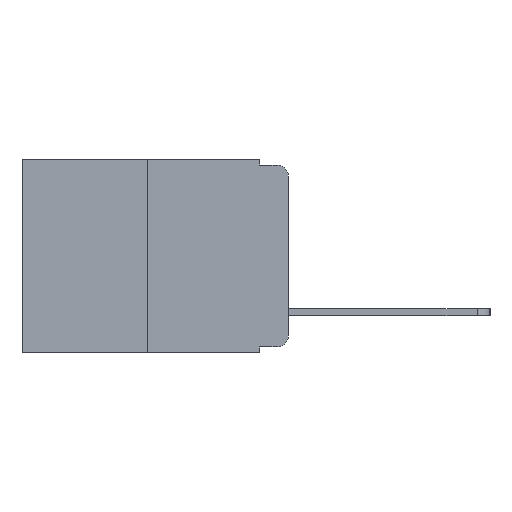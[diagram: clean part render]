
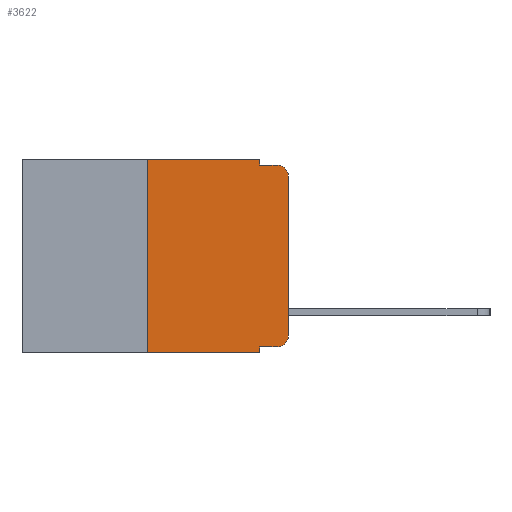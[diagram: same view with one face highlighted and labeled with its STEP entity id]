
A CAD part, left-side view. The second image highlights one B-rep face of the part: STEP entity #3622.
In plain terms, the highlighted planar face has unit normal (-1, 0, 0).
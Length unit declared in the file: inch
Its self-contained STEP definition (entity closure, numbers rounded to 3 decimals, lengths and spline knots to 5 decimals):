
#188 = LINE ( 'NONE', #12407, #15131 ) ;
#197 = CARTESIAN_POINT ( 'NONE',  ( 0., 0.02, -0.01 ) ) ;
#199 = ORIENTED_EDGE ( 'NONE', *, *, #7964, .T. ) ;
#202 = AXIS2_PLACEMENT_3D ( 'NONE', #255, #10537, #1770 ) ;
#255 = CARTESIAN_POINT ( 'NONE',  ( 0., 0.02, -0.03 ) ) ;
#1213 = EDGE_CURVE ( 'NONE', #17160, #12179, #15938, .T. ) ;
#1670 = DIRECTION ( 'NONE',  ( -1., 0., 0. ) ) ;
#1691 = EDGE_CURVE ( 'NONE', #12201, #5552, #12476, .T. ) ;
#1770 = DIRECTION ( 'NONE',  ( 0., 0., -1. ) ) ;
#1968 = ORIENTED_EDGE ( 'NONE', *, *, #8998, .F. ) ;
#2280 = ORIENTED_EDGE ( 'NONE', *, *, #17962, .T. ) ;
#2864 = EDGE_CURVE ( 'NONE', #15875, #12201, #16557, .T. ) ;
#3067 = DIRECTION ( 'NONE',  ( 0., -1., 0. ) ) ;
#3622 = ADVANCED_FACE ( 'NONE', ( #7149 ), #9745, .F. ) ;
#3859 = DIRECTION ( 'NONE',  ( 0., 0., -1. ) ) ;
#3867 = VERTEX_POINT ( 'NONE', #197 ) ;
#4126 = AXIS2_PLACEMENT_3D ( 'NONE', #13726, #9920, #9865 ) ;
#5187 = VECTOR ( 'NONE', #12238, 39.37008 ) ;
#5328 = VECTOR ( 'NONE', #7999, 39.37008 ) ;
#5380 = EDGE_CURVE ( 'NONE', #5552, #3867, #6384, .T. ) ;
#5424 = CARTESIAN_POINT ( 'NONE',  ( 0., 0.25, -0.343 ) ) ;
#5552 = VERTEX_POINT ( 'NONE', #9470 ) ;
#5699 = CARTESIAN_POINT ( 'NONE',  ( 0., 0.051, 0. ) ) ;
#5768 = ORIENTED_EDGE ( 'NONE', *, *, #1691, .F. ) ;
#5816 = CARTESIAN_POINT ( 'NONE',  ( 0., 0.02, -0.333 ) ) ;
#6181 = CARTESIAN_POINT ( 'NONE',  ( 0., 0.473, 0. ) ) ;
#6195 = ORIENTED_EDGE ( 'NONE', *, *, #9345, .T. ) ;
#6245 = ORIENTED_EDGE ( 'NONE', *, *, #5380, .F. ) ;
#6384 = LINE ( 'NONE', #17442, #13852 ) ;
#6517 = VERTEX_POINT ( 'NONE', #12123 ) ;
#6801 = CIRCLE ( 'NONE', #12951, 0.02 ) ;
#6941 = EDGE_LOOP ( 'NONE', ( #2280, #199, #6245, #5768, #10215, #1968, #10536, #10791, #6195, #10866 ) ) ;
#7149 = FACE_OUTER_BOUND ( 'NONE', #6941, .T. ) ;
#7195 = VERTEX_POINT ( 'NONE', #5816 ) ;
#7964 = EDGE_CURVE ( 'NONE', #17466, #3867, #17334, .T. ) ;
#7999 = DIRECTION ( 'NONE',  ( 0., -1., 0. ) ) ;
#8424 = LINE ( 'NONE', #9831, #15376 ) ;
#8998 = EDGE_CURVE ( 'NONE', #17160, #15875, #16871, .T. ) ;
#9116 = DIRECTION ( 'NONE',  ( 0., -1., 0. ) ) ;
#9194 = VERTEX_POINT ( 'NONE', #13927 ) ;
#9345 = EDGE_CURVE ( 'NONE', #9194, #7195, #14921, .T. ) ;
#9470 = CARTESIAN_POINT ( 'NONE',  ( 0., 0.051, -0.01 ) ) ;
#9745 = PLANE ( 'NONE',  #4126 ) ;
#9831 = CARTESIAN_POINT ( 'NONE',  ( 0., 0., 0. ) ) ;
#9865 = DIRECTION ( 'NONE',  ( 0., 0., -1. ) ) ;
#9920 = DIRECTION ( 'NONE',  ( 1., 0., 0. ) ) ;
#10076 = CARTESIAN_POINT ( 'NONE',  ( 0., 0.051, -0.333 ) ) ;
#10215 = ORIENTED_EDGE ( 'NONE', *, *, #2864, .F. ) ;
#10444 = CARTESIAN_POINT ( 'NONE',  ( 0., 0.02, -0.313 ) ) ;
#10536 = ORIENTED_EDGE ( 'NONE', *, *, #1213, .T. ) ;
#10537 = DIRECTION ( 'NONE',  ( -1., 0., 0. ) ) ;
#10791 = ORIENTED_EDGE ( 'NONE', *, *, #13660, .F. ) ;
#10856 = CARTESIAN_POINT ( 'NONE',  ( 0., 0.25, 0. ) ) ;
#10866 = ORIENTED_EDGE ( 'NONE', *, *, #14724, .T. ) ;
#11260 = DIRECTION ( 'NONE',  ( 0., 0., 1. ) ) ;
#11862 = DIRECTION ( 'NONE',  ( 0., 0., -1. ) ) ;
#12045 = VECTOR ( 'NONE', #13975, 39.37008 ) ;
#12123 = CARTESIAN_POINT ( 'NONE',  ( 0., 0., -0.313 ) ) ;
#12179 = VERTEX_POINT ( 'NONE', #16499 ) ;
#12201 = VERTEX_POINT ( 'NONE', #13752 ) ;
#12238 = DIRECTION ( 'NONE',  ( 0., 0., 1. ) ) ;
#12256 = VECTOR ( 'NONE', #3067, 39.37008 ) ;
#12407 = CARTESIAN_POINT ( 'NONE',  ( 0., 0.051, 0. ) ) ;
#12476 = LINE ( 'NONE', #5699, #12045 ) ;
#12522 = CARTESIAN_POINT ( 'NONE',  ( 0., 0.473, -0.343 ) ) ;
#12951 = AXIS2_PLACEMENT_3D ( 'NONE', #10444, #1670, #11862 ) ;
#13660 = EDGE_CURVE ( 'NONE', #9194, #12179, #188, .T. ) ;
#13726 = CARTESIAN_POINT ( 'NONE',  ( 0., 0.473, 0. ) ) ;
#13752 = CARTESIAN_POINT ( 'NONE',  ( 0., 0.051, 0. ) ) ;
#13852 = VECTOR ( 'NONE', #9116, 39.37008 ) ;
#13927 = CARTESIAN_POINT ( 'NONE',  ( 0., 0.051, -0.333 ) ) ;
#13975 = DIRECTION ( 'NONE',  ( 0., 0., -1. ) ) ;
#14216 = DIRECTION ( 'NONE',  ( 0., -1., 0. ) ) ;
#14571 = CARTESIAN_POINT ( 'NONE',  ( 0., 0.25, 0. ) ) ;
#14724 = EDGE_CURVE ( 'NONE', #7195, #6517, #6801, .T. ) ;
#14921 = LINE ( 'NONE', #10076, #17714 ) ;
#15131 = VECTOR ( 'NONE', #3859, 39.37008 ) ;
#15376 = VECTOR ( 'NONE', #11260, 39.37008 ) ;
#15875 = VERTEX_POINT ( 'NONE', #14571 ) ;
#15879 = CARTESIAN_POINT ( 'NONE',  ( 0., 0., -0.03 ) ) ;
#15938 = LINE ( 'NONE', #12522, #12256 ) ;
#16499 = CARTESIAN_POINT ( 'NONE',  ( 0., 0.051, -0.343 ) ) ;
#16557 = LINE ( 'NONE', #6181, #5328 ) ;
#16871 = LINE ( 'NONE', #10856, #5187 ) ;
#17160 = VERTEX_POINT ( 'NONE', #5424 ) ;
#17334 = CIRCLE ( 'NONE', #202, 0.02 ) ;
#17442 = CARTESIAN_POINT ( 'NONE',  ( 0., 0.051, -0.01 ) ) ;
#17466 = VERTEX_POINT ( 'NONE', #15879 ) ;
#17714 = VECTOR ( 'NONE', #14216, 39.37008 ) ;
#17962 = EDGE_CURVE ( 'NONE', #6517, #17466, #8424, .T. ) ;
